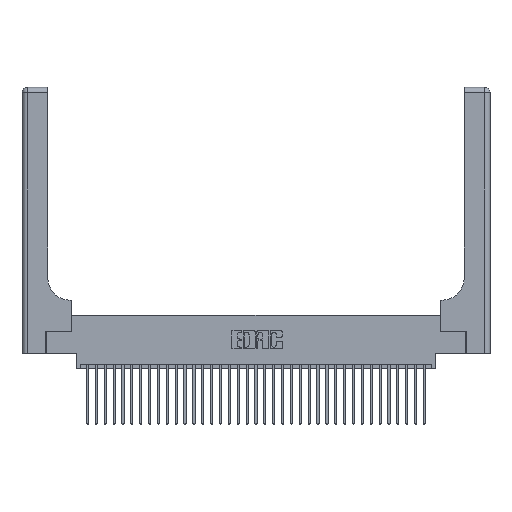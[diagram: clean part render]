
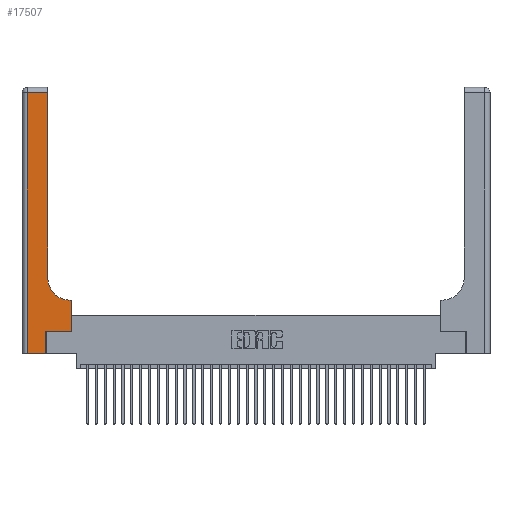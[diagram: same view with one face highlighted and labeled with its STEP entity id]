
A CAD part, top view. The second image highlights one B-rep face of the part: STEP entity #17507.
In plain terms, the highlighted planar face has unit normal (0, 0, 1).
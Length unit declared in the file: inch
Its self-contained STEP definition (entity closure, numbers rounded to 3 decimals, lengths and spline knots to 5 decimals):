
#93 = ORIENTED_EDGE ( 'NONE', *, *, #27078, .T. ) ;
#790 = VECTOR ( 'NONE', #3454, 39.37008 ) ;
#908 = CARTESIAN_POINT ( 'NONE',  ( 0.269, 0.25, 0.37 ) ) ;
#1318 = FACE_OUTER_BOUND ( 'NONE', #33552, .T. ) ;
#1679 = CIRCLE ( 'NONE', #25861, 0.25 ) ;
#2009 = CARTESIAN_POINT ( 'NONE',  ( 0.5415, 0.85, 0.37 ) ) ;
#2229 = EDGE_CURVE ( 'NONE', #31527, #24036, #35412, .T. ) ;
#2328 = EDGE_CURVE ( 'NONE', #16705, #12704, #30112, .T. ) ;
#3331 = DIRECTION ( 'NONE',  ( 0., 1., 0. ) ) ;
#3454 = DIRECTION ( 'NONE',  ( -1., 0., 0. ) ) ;
#3772 = DIRECTION ( 'NONE',  ( 1., 0., 0. ) ) ;
#3985 = ORIENTED_EDGE ( 'NONE', *, *, #2229, .T. ) ;
#4426 = DIRECTION ( 'NONE',  ( 0., 1., 0. ) ) ;
#4704 = ORIENTED_EDGE ( 'NONE', *, *, #28327, .T. ) ;
#4807 = LINE ( 'NONE', #20568, #790 ) ;
#6834 = ORIENTED_EDGE ( 'NONE', *, *, #19030, .T. ) ;
#7952 = ORIENTED_EDGE ( 'NONE', *, *, #8735, .T. ) ;
#8410 = ORIENTED_EDGE ( 'NONE', *, *, #32780, .T. ) ;
#8735 = EDGE_CURVE ( 'NONE', #24036, #34724, #15285, .T. ) ;
#9299 = LINE ( 'NONE', #908, #16334 ) ;
#10394 = CARTESIAN_POINT ( 'NONE',  ( 0.06, 3., 0.37 ) ) ;
#10506 = VERTEX_POINT ( 'NONE', #35321 ) ;
#10592 = CARTESIAN_POINT ( 'NONE',  ( 0.2915, 0.85, 0.37 ) ) ;
#10884 = CARTESIAN_POINT ( 'NONE',  ( 0.269, 0.25, 0.37 ) ) ;
#12275 = DIRECTION ( 'NONE',  ( 1., 0., 0. ) ) ;
#12704 = VERTEX_POINT ( 'NONE', #10884 ) ;
#13200 = DIRECTION ( 'NONE',  ( 0., -1., 0. ) ) ;
#13737 = EDGE_CURVE ( 'NONE', #31182, #31719, #21298, .T. ) ;
#13783 = ORIENTED_EDGE ( 'NONE', *, *, #2328, .T. ) ;
#14446 = ORIENTED_EDGE ( 'NONE', *, *, #13737, .T. ) ;
#14724 = CARTESIAN_POINT ( 'NONE',  ( 0., 0., 0.37 ) ) ;
#14996 = VECTOR ( 'NONE', #12275, 39.37008 ) ;
#15285 = LINE ( 'NONE', #29338, #34202 ) ;
#15604 = DIRECTION ( 'NONE',  ( -1., 0., 0. ) ) ;
#15729 = VECTOR ( 'NONE', #13200, 39.37008 ) ;
#16334 = VECTOR ( 'NONE', #3772, 39.37008 ) ;
#16531 = CARTESIAN_POINT ( 'NONE',  ( 0.06, 2.94, 0.37 ) ) ;
#16705 = VERTEX_POINT ( 'NONE', #30744 ) ;
#16801 = CARTESIAN_POINT ( 'NONE',  ( 0.5415, 0.6, 0.37 ) ) ;
#17297 = DIRECTION ( 'NONE',  ( 0., 0., -1. ) ) ;
#17507 = ADVANCED_FACE ( 'NONE', ( #1318 ), #34146, .F. ) ;
#17770 = DIRECTION ( 'NONE',  ( -1., 0., 0. ) ) ;
#19030 = EDGE_CURVE ( 'NONE', #30448, #31527, #1679, .T. ) ;
#20568 = CARTESIAN_POINT ( 'NONE',  ( 0.2915, 0.6, 0.37 ) ) ;
#20689 = CARTESIAN_POINT ( 'NONE',  ( 0.5585, 0.25, 0.37 ) ) ;
#21298 = LINE ( 'NONE', #20689, #27011 ) ;
#22458 = CARTESIAN_POINT ( 'NONE',  ( 0.5585, 0.6, 0.37 ) ) ;
#22710 = CARTESIAN_POINT ( 'NONE',  ( 0.269, 0., 0.37 ) ) ;
#23785 = CARTESIAN_POINT ( 'NONE',  ( 0.2915, 3., 0.37 ) ) ;
#24036 = VERTEX_POINT ( 'NONE', #28275 ) ;
#24450 = DIRECTION ( 'NONE',  ( 1., 0., 0. ) ) ;
#24988 = LINE ( 'NONE', #10394, #15729 ) ;
#25769 = CARTESIAN_POINT ( 'NONE',  ( 0., 3., 0.37 ) ) ;
#25861 = AXIS2_PLACEMENT_3D ( 'NONE', #2009, #32542, #24450 ) ;
#26547 = VECTOR ( 'NONE', #3331, 39.37008 ) ;
#26614 = EDGE_CURVE ( 'NONE', #10506, #16705, #35716, .T. ) ;
#26722 = DIRECTION ( 'NONE',  ( 0., 1., 0. ) ) ;
#27011 = VECTOR ( 'NONE', #4426, 39.37008 ) ;
#27078 = EDGE_CURVE ( 'NONE', #12704, #31182, #9299, .T. ) ;
#27916 = VECTOR ( 'NONE', #26722, 39.37008 ) ;
#28275 = CARTESIAN_POINT ( 'NONE',  ( 0.2915, 2.94, 0.37 ) ) ;
#28327 = EDGE_CURVE ( 'NONE', #31719, #30448, #4807, .T. ) ;
#29338 = CARTESIAN_POINT ( 'NONE',  ( 0., 2.94, 0.37 ) ) ;
#29611 = ORIENTED_EDGE ( 'NONE', *, *, #26614, .T. ) ;
#30112 = LINE ( 'NONE', #22710, #26547 ) ;
#30448 = VERTEX_POINT ( 'NONE', #16801 ) ;
#30744 = CARTESIAN_POINT ( 'NONE',  ( 0.269, 0., 0.37 ) ) ;
#31182 = VERTEX_POINT ( 'NONE', #31417 ) ;
#31417 = CARTESIAN_POINT ( 'NONE',  ( 0.5585, 0.25, 0.37 ) ) ;
#31527 = VERTEX_POINT ( 'NONE', #10592 ) ;
#31719 = VERTEX_POINT ( 'NONE', #22458 ) ;
#32542 = DIRECTION ( 'NONE',  ( 0., 0., -1. ) ) ;
#32780 = EDGE_CURVE ( 'NONE', #34724, #10506, #24988, .T. ) ;
#32933 = AXIS2_PLACEMENT_3D ( 'NONE', #25769, #17297, #17770 ) ;
#33552 = EDGE_LOOP ( 'NONE', ( #3985, #7952, #8410, #29611, #13783, #93, #14446, #4704, #6834 ) ) ;
#34146 = PLANE ( 'NONE',  #32933 ) ;
#34202 = VECTOR ( 'NONE', #15604, 39.37008 ) ;
#34724 = VERTEX_POINT ( 'NONE', #16531 ) ;
#35321 = CARTESIAN_POINT ( 'NONE',  ( 0.06, 0., 0.37 ) ) ;
#35412 = LINE ( 'NONE', #23785, #27916 ) ;
#35716 = LINE ( 'NONE', #14724, #14996 ) ;
